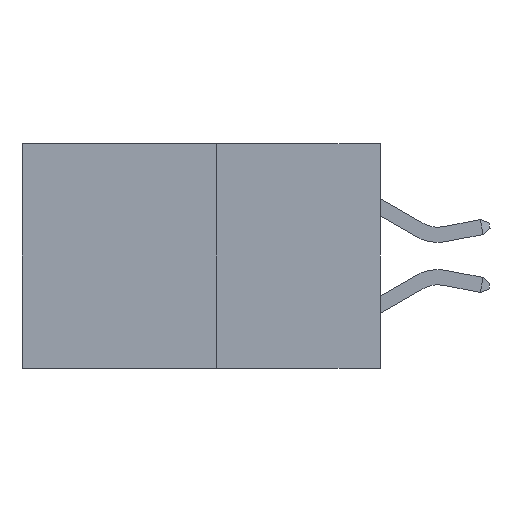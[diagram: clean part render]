
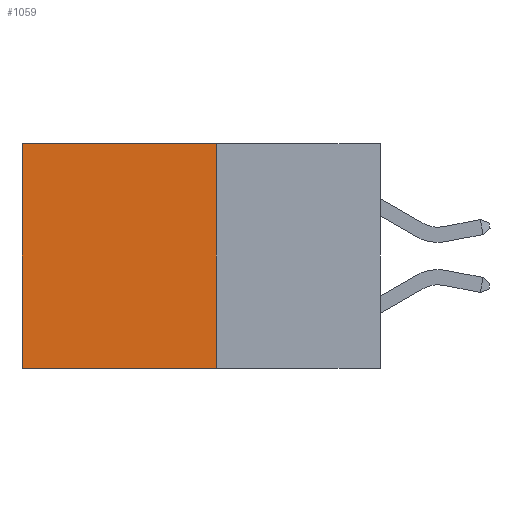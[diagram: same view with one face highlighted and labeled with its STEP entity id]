
A CAD part, left-side view. The second image highlights one B-rep face of the part: STEP entity #1059.
In plain terms, the highlighted planar face has unit normal (-1, 0, 0).
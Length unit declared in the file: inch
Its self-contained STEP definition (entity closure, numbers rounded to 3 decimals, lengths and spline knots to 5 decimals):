
#1059 = ADVANCED_FACE ( 'NONE', ( #2937 ), #9885, .F. ) ;
#1241 = EDGE_CURVE ( 'NONE', #17433, #5161, #12163, .T. ) ;
#1387 = ORIENTED_EDGE ( 'NONE', *, *, #4007, .F. ) ;
#1741 = EDGE_CURVE ( 'NONE', #19334, #2271, #18956, .T. ) ;
#2271 = VERTEX_POINT ( 'NONE', #7631 ) ;
#2937 = FACE_OUTER_BOUND ( 'NONE', #4558, .T. ) ;
#4007 = EDGE_CURVE ( 'NONE', #17433, #19334, #10984, .T. ) ;
#4558 = EDGE_LOOP ( 'NONE', ( #17187, #7956, #1387, #18869 ) ) ;
#4956 = EDGE_CURVE ( 'NONE', #5161, #2271, #19085, .T. ) ;
#5161 = VERTEX_POINT ( 'NONE', #16262 ) ;
#6015 = DIRECTION ( 'NONE',  ( 1., 0., 0. ) ) ;
#6261 = CARTESIAN_POINT ( 'NONE',  ( 0.277, 0.27, -0.37 ) ) ;
#6986 = VECTOR ( 'NONE', #11149, 39.37008 ) ;
#7533 = VECTOR ( 'NONE', #8445, 39.37008 ) ;
#7631 = CARTESIAN_POINT ( 'NONE',  ( 0.277, 0.59, -0.37 ) ) ;
#7956 = ORIENTED_EDGE ( 'NONE', *, *, #1741, .F. ) ;
#8125 = DIRECTION ( 'NONE',  ( 0., 0., -1. ) ) ;
#8445 = DIRECTION ( 'NONE',  ( 0., 1., 0. ) ) ;
#8780 = CARTESIAN_POINT ( 'NONE',  ( 0.277, 0.27, -0.37 ) ) ;
#9885 = PLANE ( 'NONE',  #12339 ) ;
#10524 = CARTESIAN_POINT ( 'NONE',  ( 0.277, 0.27, 0. ) ) ;
#10942 = CARTESIAN_POINT ( 'NONE',  ( 0.277, 0.27, 0. ) ) ;
#10984 = LINE ( 'NONE', #6261, #18398 ) ;
#11073 = CARTESIAN_POINT ( 'NONE',  ( 0.277, 0.27, -0.37 ) ) ;
#11149 = DIRECTION ( 'NONE',  ( 0., 0., -1. ) ) ;
#12163 = LINE ( 'NONE', #10942, #7533 ) ;
#12339 = AXIS2_PLACEMENT_3D ( 'NONE', #11073, #6015, #8125 ) ;
#13486 = CARTESIAN_POINT ( 'NONE',  ( 0.277, 0.59, -0.37 ) ) ;
#14844 = DIRECTION ( 'NONE',  ( 0., 0., -1. ) ) ;
#15717 = CARTESIAN_POINT ( 'NONE',  ( 0.277, 0.27, -0.37 ) ) ;
#15741 = DIRECTION ( 'NONE',  ( 0., 1., 0. ) ) ;
#16262 = CARTESIAN_POINT ( 'NONE',  ( 0.277, 0.59, 0. ) ) ;
#17187 = ORIENTED_EDGE ( 'NONE', *, *, #4956, .T. ) ;
#17433 = VERTEX_POINT ( 'NONE', #10524 ) ;
#18398 = VECTOR ( 'NONE', #14844, 39.37008 ) ;
#18477 = VECTOR ( 'NONE', #15741, 39.37008 ) ;
#18869 = ORIENTED_EDGE ( 'NONE', *, *, #1241, .T. ) ;
#18956 = LINE ( 'NONE', #15717, #18477 ) ;
#19085 = LINE ( 'NONE', #13486, #6986 ) ;
#19334 = VERTEX_POINT ( 'NONE', #8780 ) ;
